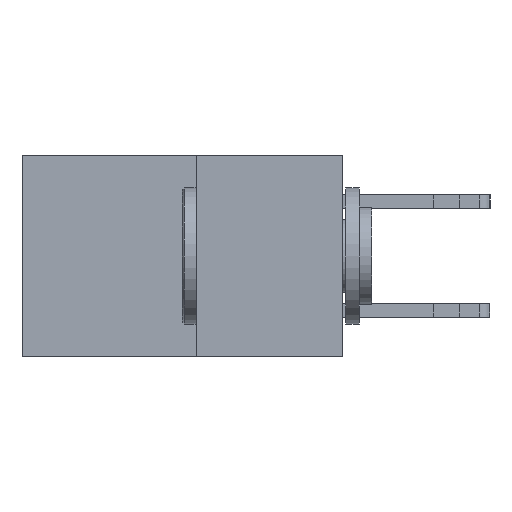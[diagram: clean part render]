
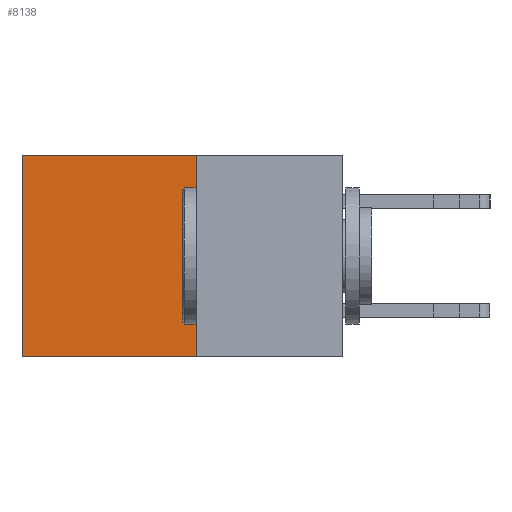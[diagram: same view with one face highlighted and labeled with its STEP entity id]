
A CAD part, left-side view. The second image highlights one B-rep face of the part: STEP entity #8138.
In plain terms, the highlighted planar face has unit normal (-1, 0, 0).
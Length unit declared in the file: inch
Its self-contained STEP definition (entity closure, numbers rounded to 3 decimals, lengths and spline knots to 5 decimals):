
#78 = DIRECTION ( 'NONE',  ( 0., 0., -1. ) ) ;
#1541 = CARTESIAN_POINT ( 'NONE',  ( 0.277, 0.27, 0. ) ) ;
#2239 = CARTESIAN_POINT ( 'NONE',  ( 0.277, 0.27, -0.37 ) ) ;
#3321 = ORIENTED_EDGE ( 'NONE', *, *, #19783, .F. ) ;
#4181 = VERTEX_POINT ( 'NONE', #22097 ) ;
#5419 = LINE ( 'NONE', #9773, #6145 ) ;
#5969 = DIRECTION ( 'NONE',  ( 0., 1., 0. ) ) ;
#6145 = VECTOR ( 'NONE', #25832, 39.37008 ) ;
#6584 = DIRECTION ( 'NONE',  ( 0., 1., 0. ) ) ;
#6877 = DIRECTION ( 'NONE',  ( 0., 0., -1. ) ) ;
#8138 = ADVANCED_FACE ( 'NONE', ( #25273 ), #11443, .F. ) ;
#8609 = VECTOR ( 'NONE', #6584, 39.37008 ) ;
#8684 = CARTESIAN_POINT ( 'NONE',  ( 0.277, 0.27, -0.37 ) ) ;
#8881 = ORIENTED_EDGE ( 'NONE', *, *, #9570, .F. ) ;
#9155 = AXIS2_PLACEMENT_3D ( 'NONE', #2239, #13722, #78 ) ;
#9570 = EDGE_CURVE ( 'NONE', #17579, #11329, #5419, .T. ) ;
#9773 = CARTESIAN_POINT ( 'NONE',  ( 0.277, 0.27, -0.37 ) ) ;
#10522 = CARTESIAN_POINT ( 'NONE',  ( 0.277, 0.27, 0. ) ) ;
#11329 = VERTEX_POINT ( 'NONE', #8684 ) ;
#11379 = VECTOR ( 'NONE', #6877, 39.37008 ) ;
#11443 = PLANE ( 'NONE',  #9155 ) ;
#11576 = EDGE_LOOP ( 'NONE', ( #27414, #3321, #8881, #15121 ) ) ;
#12433 = VERTEX_POINT ( 'NONE', #16078 ) ;
#13722 = DIRECTION ( 'NONE',  ( 1., 0., 0. ) ) ;
#14724 = VECTOR ( 'NONE', #5969, 39.37008 ) ;
#14785 = EDGE_CURVE ( 'NONE', #17579, #4181, #26938, .T. ) ;
#15121 = ORIENTED_EDGE ( 'NONE', *, *, #14785, .T. ) ;
#16078 = CARTESIAN_POINT ( 'NONE',  ( 0.277, 0.59, -0.37 ) ) ;
#17579 = VERTEX_POINT ( 'NONE', #1541 ) ;
#17752 = EDGE_CURVE ( 'NONE', #4181, #12433, #27504, .T. ) ;
#19783 = EDGE_CURVE ( 'NONE', #11329, #12433, #21544, .T. ) ;
#20245 = CARTESIAN_POINT ( 'NONE',  ( 0.277, 0.27, -0.37 ) ) ;
#20646 = CARTESIAN_POINT ( 'NONE',  ( 0.277, 0.59, -0.37 ) ) ;
#21544 = LINE ( 'NONE', #20245, #8609 ) ;
#22097 = CARTESIAN_POINT ( 'NONE',  ( 0.277, 0.59, 0. ) ) ;
#25273 = FACE_OUTER_BOUND ( 'NONE', #11576, .T. ) ;
#25832 = DIRECTION ( 'NONE',  ( 0., 0., -1. ) ) ;
#26938 = LINE ( 'NONE', #10522, #14724 ) ;
#27414 = ORIENTED_EDGE ( 'NONE', *, *, #17752, .T. ) ;
#27504 = LINE ( 'NONE', #20646, #11379 ) ;
